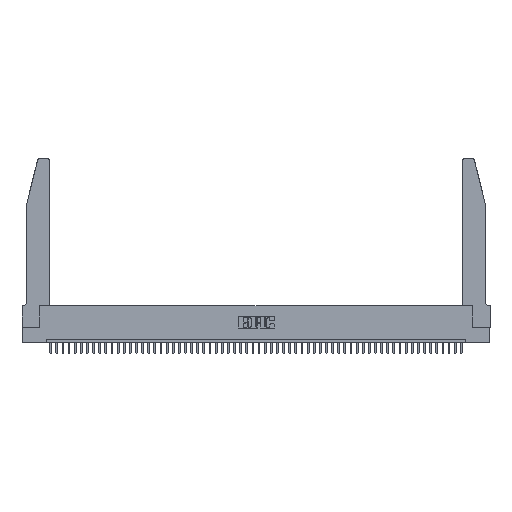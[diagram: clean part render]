
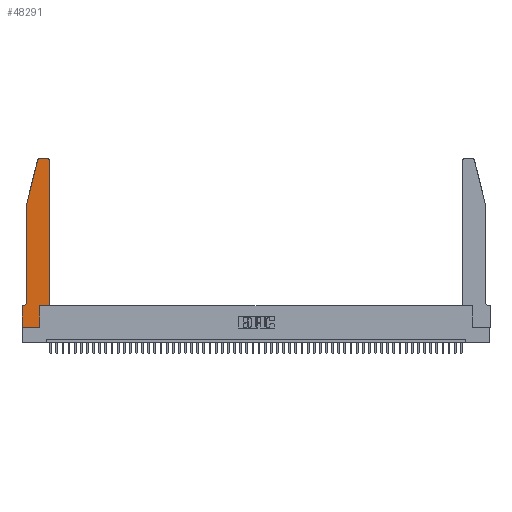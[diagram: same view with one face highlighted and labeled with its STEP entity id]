
A CAD part, top view. The second image highlights one B-rep face of the part: STEP entity #48291.
In plain terms, the highlighted planar face has unit normal (0, 0, 1).
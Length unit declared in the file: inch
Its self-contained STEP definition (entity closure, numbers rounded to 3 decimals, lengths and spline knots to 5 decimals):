
#1387 = CARTESIAN_POINT ( 'NONE',  ( 0., 0.35, 0.37 ) ) ;
#1875 = LINE ( 'NONE', #30630, #7018 ) ;
#2764 = CARTESIAN_POINT ( 'NONE',  ( 0.2865, 0.35, 0.37 ) ) ;
#3296 = EDGE_CURVE ( 'NONE', #13504, #36583, #39664, .T. ) ;
#3637 = VERTEX_POINT ( 'NONE', #22300 ) ;
#4108 = CARTESIAN_POINT ( 'NONE',  ( 0.284, 2.72, 0.37 ) ) ;
#4590 = EDGE_LOOP ( 'NONE', ( #19668, #40346, #16007, #42620, #14873, #36247, #47508, #15574, #51293, #9095, #41233, #46263 ) ) ;
#4647 = DIRECTION ( 'NONE',  ( 0., 0., -1. ) ) ;
#5646 = CARTESIAN_POINT ( 'NONE',  ( 0., 0.35, 0.37 ) ) ;
#5986 = AXIS2_PLACEMENT_3D ( 'NONE', #5646, #33638, #49985 ) ;
#6172 = CIRCLE ( 'NONE', #20499, 0.07 ) ;
#6407 = DIRECTION ( 'NONE',  ( 1., 0., 0. ) ) ;
#6667 = CARTESIAN_POINT ( 'NONE',  ( 0.0755, 2., 0.37 ) ) ;
#7018 = VECTOR ( 'NONE', #6407, 39.37008 ) ;
#9095 = ORIENTED_EDGE ( 'NONE', *, *, #3296, .T. ) ;
#9795 = VERTEX_POINT ( 'NONE', #28459 ) ;
#9988 = LINE ( 'NONE', #23225, #11949 ) ;
#10182 = VERTEX_POINT ( 'NONE', #21922 ) ;
#11382 = VERTEX_POINT ( 'NONE', #14292 ) ;
#11788 = VECTOR ( 'NONE', #29222, 39.37008 ) ;
#11949 = VECTOR ( 'NONE', #31627, 39.37008 ) ;
#12983 = LINE ( 'NONE', #36347, #11788 ) ;
#13504 = VERTEX_POINT ( 'NONE', #2764 ) ;
#13594 = DIRECTION ( 'NONE',  ( 1., 0., 0. ) ) ;
#14292 = CARTESIAN_POINT ( 'NONE',  ( 0.0055, 0.35, 0.37 ) ) ;
#14873 = ORIENTED_EDGE ( 'NONE', *, *, #40147, .T. ) ;
#14881 = EDGE_CURVE ( 'NONE', #33128, #27750, #43278, .T. ) ;
#15045 = CARTESIAN_POINT ( 'NONE',  ( 0.0755, 0.35, 0.37 ) ) ;
#15574 = ORIENTED_EDGE ( 'NONE', *, *, #15580, .T. ) ;
#15580 = EDGE_CURVE ( 'NONE', #3637, #32304, #1875, .T. ) ;
#16007 = ORIENTED_EDGE ( 'NONE', *, *, #44563, .T. ) ;
#16411 = DIRECTION ( 'NONE',  ( 1., 0., 0. ) ) ;
#17563 = EDGE_CURVE ( 'NONE', #20114, #3637, #32239, .T. ) ;
#17789 = CARTESIAN_POINT ( 'NONE',  ( 0.4505, 0.35, 0.37 ) ) ;
#19668 = ORIENTED_EDGE ( 'NONE', *, *, #52248, .T. ) ;
#19737 = DIRECTION ( 'NONE',  ( -1., 0., 0. ) ) ;
#20114 = VERTEX_POINT ( 'NONE', #1387 ) ;
#20499 = AXIS2_PLACEMENT_3D ( 'NONE', #33481, #4647, #49326 ) ;
#21189 = VECTOR ( 'NONE', #27171, 39.37008 ) ;
#21359 = CARTESIAN_POINT ( 'NONE',  ( 0.25487, 2.72718, 0.37 ) ) ;
#21824 = DIRECTION ( 'NONE',  ( 1., 0., 0. ) ) ;
#21922 = CARTESIAN_POINT ( 'NONE',  ( 0.4505, 2.72, 0.37 ) ) ;
#22276 = CIRCLE ( 'NONE', #46775, 0.03 ) ;
#22300 = CARTESIAN_POINT ( 'NONE',  ( 0., 0., 0.37 ) ) ;
#22408 = LINE ( 'NONE', #15045, #32041 ) ;
#22440 = VERTEX_POINT ( 'NONE', #6667 ) ;
#22733 = VECTOR ( 'NONE', #46625, 39.37008 ) ;
#23225 = CARTESIAN_POINT ( 'NONE',  ( 0.0755, 2., 0.37 ) ) ;
#23639 = FACE_OUTER_BOUND ( 'NONE', #4590, .T. ) ;
#23997 = AXIS2_PLACEMENT_3D ( 'NONE', #4108, #36361, #16411 ) ;
#24303 = LINE ( 'NONE', #26079, #48527 ) ;
#25364 = DIRECTION ( 'NONE',  ( -1., 0., 0. ) ) ;
#25858 = LINE ( 'NONE', #50528, #22733 ) ;
#26079 = CARTESIAN_POINT ( 'NONE',  ( 0.2605, 2.75, 0.37 ) ) ;
#27171 = DIRECTION ( 'NONE',  ( 0., 1., 0. ) ) ;
#27750 = VERTEX_POINT ( 'NONE', #21359 ) ;
#28388 = CARTESIAN_POINT ( 'NONE',  ( 0.2865, 0., 0.37 ) ) ;
#28459 = CARTESIAN_POINT ( 'NONE',  ( 0.0755, 0.42, 0.37 ) ) ;
#29222 = DIRECTION ( 'NONE',  ( 0., 1., 0. ) ) ;
#30630 = CARTESIAN_POINT ( 'NONE',  ( 0., 0., 0.37 ) ) ;
#31627 = DIRECTION ( 'NONE',  ( 0., -1., 0. ) ) ;
#32041 = VECTOR ( 'NONE', #19737, 39.37008 ) ;
#32239 = LINE ( 'NONE', #50091, #34056 ) ;
#32304 = VERTEX_POINT ( 'NONE', #28388 ) ;
#33128 = VERTEX_POINT ( 'NONE', #46467 ) ;
#33481 = CARTESIAN_POINT ( 'NONE',  ( 0.0055, 0.42, 0.37 ) ) ;
#33638 = DIRECTION ( 'NONE',  ( 0., 0., 1. ) ) ;
#34056 = VECTOR ( 'NONE', #41890, 39.37008 ) ;
#34560 = CARTESIAN_POINT ( 'NONE',  ( 0.4505, 0.35, 0.37 ) ) ;
#34750 = EDGE_CURVE ( 'NONE', #36583, #10182, #12983, .T. ) ;
#34935 = CARTESIAN_POINT ( 'NONE',  ( 0.4205, 2.75, 0.37 ) ) ;
#36247 = ORIENTED_EDGE ( 'NONE', *, *, #51826, .T. ) ;
#36347 = CARTESIAN_POINT ( 'NONE',  ( 0.4505, 0.35, 0.37 ) ) ;
#36361 = DIRECTION ( 'NONE',  ( 0., 0., 1. ) ) ;
#36583 = VERTEX_POINT ( 'NONE', #34560 ) ;
#36600 = VERTEX_POINT ( 'NONE', #34935 ) ;
#37711 = CARTESIAN_POINT ( 'NONE',  ( 0.4205, 2.72, 0.37 ) ) ;
#39664 = LINE ( 'NONE', #17789, #48624 ) ;
#40147 = EDGE_CURVE ( 'NONE', #9795, #11382, #6172, .T. ) ;
#40346 = ORIENTED_EDGE ( 'NONE', *, *, #14881, .T. ) ;
#41233 = ORIENTED_EDGE ( 'NONE', *, *, #34750, .T. ) ;
#41890 = DIRECTION ( 'NONE',  ( 0., -1., 0. ) ) ;
#42620 = ORIENTED_EDGE ( 'NONE', *, *, #49203, .T. ) ;
#42924 = LINE ( 'NONE', #51542, #21189 ) ;
#43278 = CIRCLE ( 'NONE', #23997, 0.03 ) ;
#44563 = EDGE_CURVE ( 'NONE', #27750, #22440, #25858, .T. ) ;
#46066 = DIRECTION ( 'NONE',  ( 0., 0., 1. ) ) ;
#46263 = ORIENTED_EDGE ( 'NONE', *, *, #48359, .T. ) ;
#46313 = EDGE_CURVE ( 'NONE', #32304, #13504, #42924, .T. ) ;
#46467 = CARTESIAN_POINT ( 'NONE',  ( 0.284, 2.75, 0.37 ) ) ;
#46625 = DIRECTION ( 'NONE',  ( -0.239, -0.971, 0. ) ) ;
#46775 = AXIS2_PLACEMENT_3D ( 'NONE', #37711, #46066, #13594 ) ;
#47508 = ORIENTED_EDGE ( 'NONE', *, *, #17563, .T. ) ;
#48291 = ADVANCED_FACE ( 'NONE', ( #23639 ), #49618, .T. ) ;
#48359 = EDGE_CURVE ( 'NONE', #10182, #36600, #22276, .T. ) ;
#48527 = VECTOR ( 'NONE', #25364, 39.37008 ) ;
#48624 = VECTOR ( 'NONE', #21824, 39.37008 ) ;
#49203 = EDGE_CURVE ( 'NONE', #22440, #9795, #9988, .T. ) ;
#49326 = DIRECTION ( 'NONE',  ( -1., 0., 0. ) ) ;
#49618 = PLANE ( 'NONE',  #5986 ) ;
#49985 = DIRECTION ( 'NONE',  ( 1., 0., 0. ) ) ;
#50091 = CARTESIAN_POINT ( 'NONE',  ( 0., 0., 0.37 ) ) ;
#50528 = CARTESIAN_POINT ( 'NONE',  ( 0.0755, 2., 0.37 ) ) ;
#51293 = ORIENTED_EDGE ( 'NONE', *, *, #46313, .T. ) ;
#51542 = CARTESIAN_POINT ( 'NONE',  ( 0.2865, 0.35, 0.37 ) ) ;
#51826 = EDGE_CURVE ( 'NONE', #11382, #20114, #22408, .T. ) ;
#52248 = EDGE_CURVE ( 'NONE', #36600, #33128, #24303, .T. ) ;
